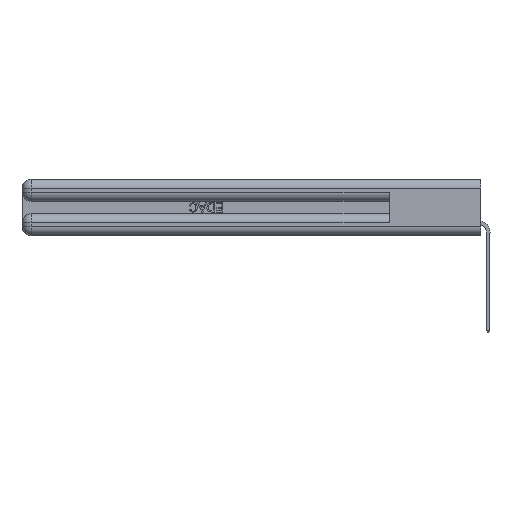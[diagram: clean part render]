
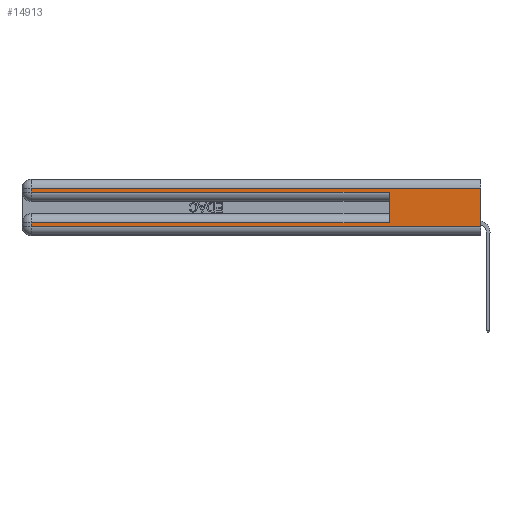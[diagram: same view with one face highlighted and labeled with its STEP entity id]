
A CAD part, left-side view. The second image highlights one B-rep face of the part: STEP entity #14913.
In plain terms, the highlighted planar face has unit normal (-1, 0, 0).
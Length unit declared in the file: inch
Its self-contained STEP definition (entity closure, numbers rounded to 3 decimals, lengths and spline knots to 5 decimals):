
#167 = DIRECTION ( 'NONE',  ( 0., -1., 0. ) ) ;
#170 = VERTEX_POINT ( 'NONE', #2117 ) ;
#179 = VECTOR ( 'NONE', #6713, 39.37008 ) ;
#994 = DIRECTION ( 'NONE',  ( 0., 0., -1. ) ) ;
#1685 = ORIENTED_EDGE ( 'NONE', *, *, #14375, .T. ) ;
#2007 = EDGE_CURVE ( 'NONE', #13266, #18064, #9613, .T. ) ;
#2117 = CARTESIAN_POINT ( 'NONE',  ( 0., 0.6, 0.285 ) ) ;
#2362 = LINE ( 'NONE', #11907, #7550 ) ;
#2597 = VERTEX_POINT ( 'NONE', #6983 ) ;
#2765 = VECTOR ( 'NONE', #17836, 39.37008 ) ;
#3400 = ORIENTED_EDGE ( 'NONE', *, *, #10743, .T. ) ;
#3916 = ORIENTED_EDGE ( 'NONE', *, *, #10871, .F. ) ;
#3997 = VERTEX_POINT ( 'NONE', #10589 ) ;
#4044 = ORIENTED_EDGE ( 'NONE', *, *, #32033, .T. ) ;
#4204 = CARTESIAN_POINT ( 'NONE',  ( 0., 0., 0.085 ) ) ;
#4334 = DIRECTION ( 'NONE',  ( 1., 0., 0. ) ) ;
#4643 = LINE ( 'NONE', #13208, #29030 ) ;
#4723 = EDGE_LOOP ( 'NONE', ( #3916, #19496, #4044, #1685, #30492, #26928, #3400, #18081 ) ) ;
#5658 = CARTESIAN_POINT ( 'NONE',  ( 0., 2.94, 0.285 ) ) ;
#6713 = DIRECTION ( 'NONE',  ( 0., 0., 1. ) ) ;
#6928 = DIRECTION ( 'NONE',  ( 0., 0., -1. ) ) ;
#6983 = CARTESIAN_POINT ( 'NONE',  ( 0., 2.94, 0.06 ) ) ;
#7550 = VECTOR ( 'NONE', #6928, 39.37008 ) ;
#8076 = CARTESIAN_POINT ( 'NONE',  ( 0., 2.94, 0.085 ) ) ;
#8691 = EDGE_CURVE ( 'NONE', #3997, #170, #28562, .T. ) ;
#9287 = VECTOR ( 'NONE', #27249, 39.37008 ) ;
#9316 = VECTOR ( 'NONE', #994, 39.37008 ) ;
#9379 = CARTESIAN_POINT ( 'NONE',  ( 0., 0., 0.37 ) ) ;
#9410 = CARTESIAN_POINT ( 'NONE',  ( 0., 0.6, 0.145 ) ) ;
#9613 = LINE ( 'NONE', #27108, #2765 ) ;
#9688 = LINE ( 'NONE', #11914, #9287 ) ;
#10589 = CARTESIAN_POINT ( 'NONE',  ( 0., 0.6, 0.085 ) ) ;
#10743 = EDGE_CURVE ( 'NONE', #24726, #2597, #19292, .T. ) ;
#10871 = EDGE_CURVE ( 'NONE', #13266, #13379, #28429, .T. ) ;
#11209 = EDGE_CURVE ( 'NONE', #2597, #13379, #9688, .T. ) ;
#11728 = VERTEX_POINT ( 'NONE', #5658 ) ;
#11907 = CARTESIAN_POINT ( 'NONE',  ( 0., 2.94, 0.37 ) ) ;
#11914 = CARTESIAN_POINT ( 'NONE',  ( 0., 0., 0.06 ) ) ;
#12983 = FACE_OUTER_BOUND ( 'NONE', #4723, .T. ) ;
#13208 = CARTESIAN_POINT ( 'NONE',  ( 0., 0., 0.285 ) ) ;
#13266 = VERTEX_POINT ( 'NONE', #27936 ) ;
#13379 = VERTEX_POINT ( 'NONE', #28588 ) ;
#13803 = EDGE_CURVE ( 'NONE', #3997, #24726, #30288, .T. ) ;
#14375 = EDGE_CURVE ( 'NONE', #11728, #170, #4643, .T. ) ;
#14913 = ADVANCED_FACE ( 'NONE', ( #12983 ), #30236, .F. ) ;
#15567 = DIRECTION ( 'NONE',  ( 0., 0., -1. ) ) ;
#15637 = AXIS2_PLACEMENT_3D ( 'NONE', #9379, #4334, #15567 ) ;
#16115 = VECTOR ( 'NONE', #16882, 39.37008 ) ;
#16882 = DIRECTION ( 'NONE',  ( 0., 0., -1. ) ) ;
#17836 = DIRECTION ( 'NONE',  ( 0., 1., 0. ) ) ;
#18064 = VERTEX_POINT ( 'NONE', #21730 ) ;
#18081 = ORIENTED_EDGE ( 'NONE', *, *, #11209, .T. ) ;
#19292 = LINE ( 'NONE', #29148, #9316 ) ;
#19496 = ORIENTED_EDGE ( 'NONE', *, *, #2007, .T. ) ;
#21730 = CARTESIAN_POINT ( 'NONE',  ( 0., 2.94, 0.31 ) ) ;
#24726 = VERTEX_POINT ( 'NONE', #8076 ) ;
#26928 = ORIENTED_EDGE ( 'NONE', *, *, #13803, .T. ) ;
#27108 = CARTESIAN_POINT ( 'NONE',  ( 0., 0., 0.31 ) ) ;
#27249 = DIRECTION ( 'NONE',  ( 0., -1., 0. ) ) ;
#27936 = CARTESIAN_POINT ( 'NONE',  ( 0., 0., 0.31 ) ) ;
#28429 = LINE ( 'NONE', #29587, #16115 ) ;
#28562 = LINE ( 'NONE', #9410, #179 ) ;
#28588 = CARTESIAN_POINT ( 'NONE',  ( 0., 0., 0.06 ) ) ;
#29030 = VECTOR ( 'NONE', #167, 39.37008 ) ;
#29148 = CARTESIAN_POINT ( 'NONE',  ( 0., 2.94, 0.37 ) ) ;
#29587 = CARTESIAN_POINT ( 'NONE',  ( 0., 0., 0.37 ) ) ;
#29893 = DIRECTION ( 'NONE',  ( 0., 1., 0. ) ) ;
#30236 = PLANE ( 'NONE',  #15637 ) ;
#30288 = LINE ( 'NONE', #4204, #30665 ) ;
#30492 = ORIENTED_EDGE ( 'NONE', *, *, #8691, .F. ) ;
#30665 = VECTOR ( 'NONE', #29893, 39.37008 ) ;
#32033 = EDGE_CURVE ( 'NONE', #18064, #11728, #2362, .T. ) ;
